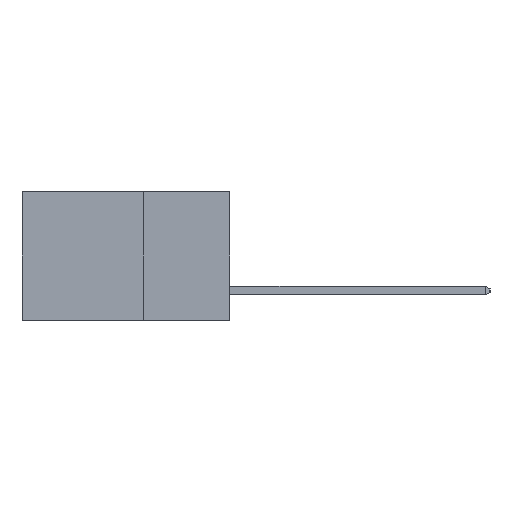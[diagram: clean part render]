
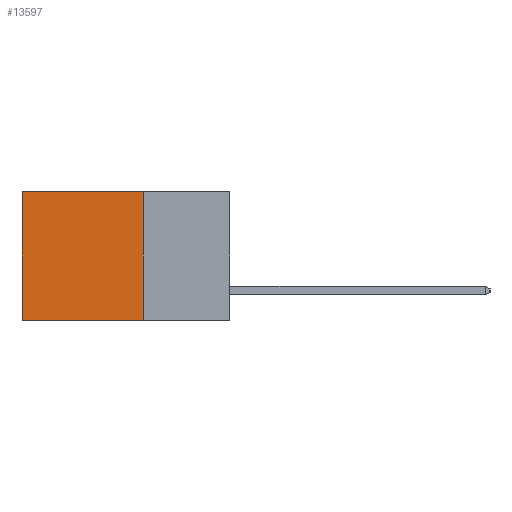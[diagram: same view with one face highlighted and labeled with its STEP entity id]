
A CAD part, left-side view. The second image highlights one B-rep face of the part: STEP entity #13597.
In plain terms, the highlighted planar face has unit normal (-1, 0, 0).
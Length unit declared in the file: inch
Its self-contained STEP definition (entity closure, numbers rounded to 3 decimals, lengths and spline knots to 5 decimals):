
#131 = LINE ( 'NONE', #7660, #6115 ) ;
#540 = CARTESIAN_POINT ( 'NONE',  ( 0.298, 0.6, -0.37 ) ) ;
#996 = EDGE_CURVE ( 'NONE', #8018, #5889, #8072, .T. ) ;
#1002 = CARTESIAN_POINT ( 'NONE',  ( 0.298, 0.25, 0. ) ) ;
#1409 = DIRECTION ( 'NONE',  ( 0., 0., -1. ) ) ;
#1920 = CARTESIAN_POINT ( 'NONE',  ( 0.298, 0.6, 0. ) ) ;
#1948 = EDGE_LOOP ( 'NONE', ( #9096, #5227, #4904, #11973 ) ) ;
#2257 = DIRECTION ( 'NONE',  ( 0., 0., -1. ) ) ;
#4904 = ORIENTED_EDGE ( 'NONE', *, *, #8666, .F. ) ;
#5117 = DIRECTION ( 'NONE',  ( 0., 0., -1. ) ) ;
#5227 = ORIENTED_EDGE ( 'NONE', *, *, #996, .F. ) ;
#5447 = DIRECTION ( 'NONE',  ( 0., 1., 0. ) ) ;
#5629 = EDGE_CURVE ( 'NONE', #8800, #5889, #10623, .T. ) ;
#5889 = VERTEX_POINT ( 'NONE', #540 ) ;
#6115 = VECTOR ( 'NONE', #5447, 39.37008 ) ;
#6114 = CARTESIAN_POINT ( 'NONE',  ( 0.298, 0.25, 0. ) ) ;
#7660 = CARTESIAN_POINT ( 'NONE',  ( 0.298, 0.25, 0. ) ) ;
#7747 = AXIS2_PLACEMENT_3D ( 'NONE', #1002, #9124, #2257 ) ;
#7779 = VECTOR ( 'NONE', #1409, 39.37008 ) ;
#8018 = VERTEX_POINT ( 'NONE', #10243 ) ;
#8072 = LINE ( 'NONE', #10103, #13209 ) ;
#8666 = EDGE_CURVE ( 'NONE', #13277, #8018, #14327, .T. ) ;
#8800 = VERTEX_POINT ( 'NONE', #12869 ) ;
#9096 = ORIENTED_EDGE ( 'NONE', *, *, #5629, .T. ) ;
#9124 = DIRECTION ( 'NONE',  ( 1., 0., 0. ) ) ;
#9594 = FACE_OUTER_BOUND ( 'NONE', #1948, .T. ) ;
#10103 = CARTESIAN_POINT ( 'NONE',  ( 0.298, 0.25, -0.37 ) ) ;
#10243 = CARTESIAN_POINT ( 'NONE',  ( 0.298, 0.25, -0.37 ) ) ;
#10623 = LINE ( 'NONE', #1920, #7779 ) ;
#10881 = DIRECTION ( 'NONE',  ( 0., 1., 0. ) ) ;
#11307 = EDGE_CURVE ( 'NONE', #13277, #8800, #131, .T. ) ;
#11599 = VECTOR ( 'NONE', #5117, 39.37008 ) ;
#11973 = ORIENTED_EDGE ( 'NONE', *, *, #11307, .T. ) ;
#12696 = CARTESIAN_POINT ( 'NONE',  ( 0.298, 0.25, 0. ) ) ;
#12869 = CARTESIAN_POINT ( 'NONE',  ( 0.298, 0.6, 0. ) ) ;
#13209 = VECTOR ( 'NONE', #10881, 39.37008 ) ;
#13277 = VERTEX_POINT ( 'NONE', #6114 ) ;
#13597 = ADVANCED_FACE ( 'NONE', ( #9594 ), #14285, .F. ) ;
#14285 = PLANE ( 'NONE',  #7747 ) ;
#14327 = LINE ( 'NONE', #12696, #11599 ) ;
